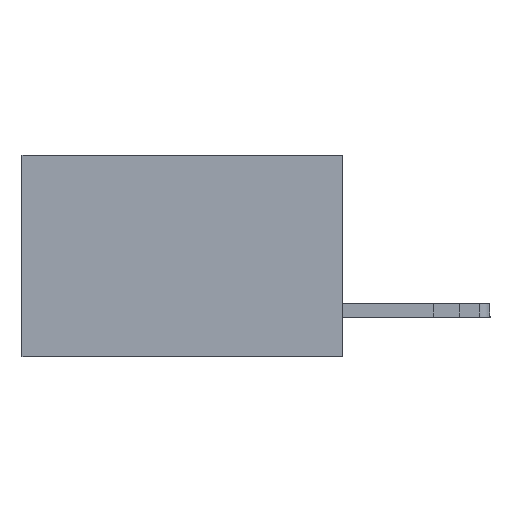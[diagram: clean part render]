
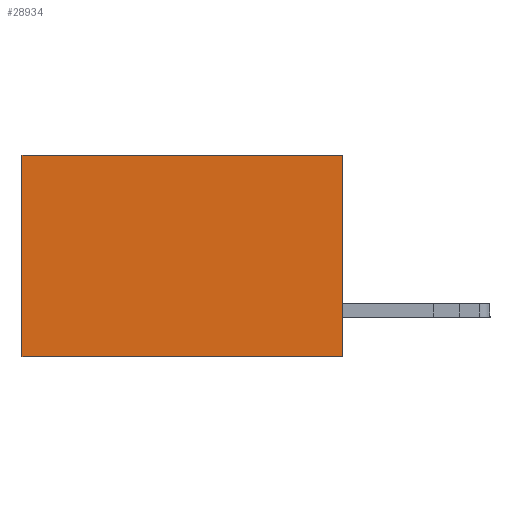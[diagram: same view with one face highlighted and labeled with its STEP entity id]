
A CAD part, left-side view. The second image highlights one B-rep face of the part: STEP entity #28934.
In plain terms, the highlighted planar face has unit normal (-1, 0, 0).
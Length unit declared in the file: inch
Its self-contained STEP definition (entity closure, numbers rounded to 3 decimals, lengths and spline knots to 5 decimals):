
#344 = VERTEX_POINT ( 'NONE', #26593 ) ;
#2467 = DIRECTION ( 'NONE',  ( 0., 1., 0. ) ) ;
#2763 = LINE ( 'NONE', #7867, #14792 ) ;
#3814 = AXIS2_PLACEMENT_3D ( 'NONE', #25109, #10802, #27491 ) ;
#4690 = LINE ( 'NONE', #14470, #17456 ) ;
#5344 = ORIENTED_EDGE ( 'NONE', *, *, #19220, .T. ) ;
#5836 = ORIENTED_EDGE ( 'NONE', *, *, #13358, .F. ) ;
#5985 = PLANE ( 'NONE',  #3814 ) ;
#6717 = VERTEX_POINT ( 'NONE', #17670 ) ;
#7867 = CARTESIAN_POINT ( 'NONE',  ( 0.277, 0., -0.37 ) ) ;
#9487 = LINE ( 'NONE', #27923, #27753 ) ;
#10284 = DIRECTION ( 'NONE',  ( 0., 0., -1. ) ) ;
#10802 = DIRECTION ( 'NONE',  ( 1., 0., 0. ) ) ;
#13358 = EDGE_CURVE ( 'NONE', #344, #24183, #2763, .T. ) ;
#14470 = CARTESIAN_POINT ( 'NONE',  ( 0.277, 0., -0.37 ) ) ;
#14792 = VECTOR ( 'NONE', #10284, 39.37008 ) ;
#15237 = CARTESIAN_POINT ( 'NONE',  ( 0.277, 0.59, -0.37 ) ) ;
#17443 = VERTEX_POINT ( 'NONE', #20891 ) ;
#17456 = VECTOR ( 'NONE', #2467, 39.37008 ) ;
#17647 = DIRECTION ( 'NONE',  ( 0., 0., -1. ) ) ;
#17670 = CARTESIAN_POINT ( 'NONE',  ( 0.277, 0.59, -0.37 ) ) ;
#19220 = EDGE_CURVE ( 'NONE', #17443, #6717, #27851, .T. ) ;
#19634 = CARTESIAN_POINT ( 'NONE',  ( 0.277, 0., -0.37 ) ) ;
#20427 = FACE_OUTER_BOUND ( 'NONE', #27075, .T. ) ;
#20891 = CARTESIAN_POINT ( 'NONE',  ( 0.277, 0.59, 0. ) ) ;
#21578 = VECTOR ( 'NONE', #17647, 39.37008 ) ;
#21620 = EDGE_CURVE ( 'NONE', #344, #17443, #9487, .T. ) ;
#24183 = VERTEX_POINT ( 'NONE', #19634 ) ;
#25109 = CARTESIAN_POINT ( 'NONE',  ( 0.277, 0., -0.37 ) ) ;
#26049 = ORIENTED_EDGE ( 'NONE', *, *, #28641, .F. ) ;
#26593 = CARTESIAN_POINT ( 'NONE',  ( 0.277, 0., 0. ) ) ;
#27075 = EDGE_LOOP ( 'NONE', ( #5344, #26049, #5836, #27487 ) ) ;
#27487 = ORIENTED_EDGE ( 'NONE', *, *, #21620, .T. ) ;
#27491 = DIRECTION ( 'NONE',  ( 0., 0., -1. ) ) ;
#27753 = VECTOR ( 'NONE', #30295, 39.37008 ) ;
#27851 = LINE ( 'NONE', #15237, #21578 ) ;
#27923 = CARTESIAN_POINT ( 'NONE',  ( 0.277, 0., 0. ) ) ;
#28641 = EDGE_CURVE ( 'NONE', #24183, #6717, #4690, .T. ) ;
#28934 = ADVANCED_FACE ( 'NONE', ( #20427 ), #5985, .F. ) ;
#30295 = DIRECTION ( 'NONE',  ( 0., 1., 0. ) ) ;
